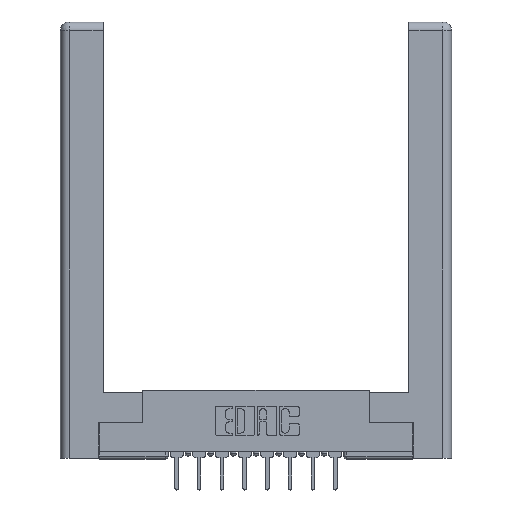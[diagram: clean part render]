
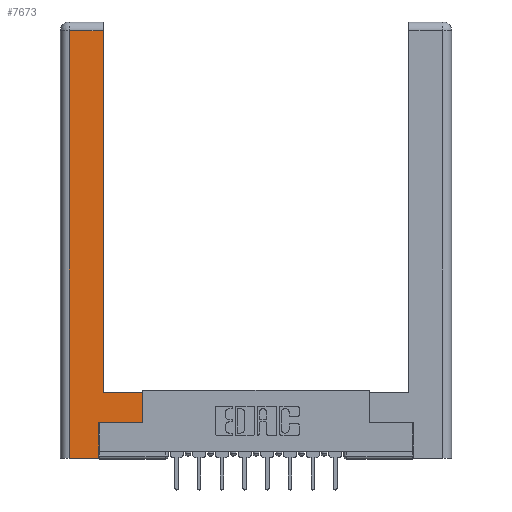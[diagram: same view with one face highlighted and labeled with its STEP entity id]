
A CAD part, top view. The second image highlights one B-rep face of the part: STEP entity #7673.
In plain terms, the highlighted planar face has unit normal (0, 0, 1).
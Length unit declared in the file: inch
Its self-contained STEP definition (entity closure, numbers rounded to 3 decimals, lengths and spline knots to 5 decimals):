
#47 = ORIENTED_EDGE ( 'NONE', *, *, #10888, .T. ) ;
#483 = VECTOR ( 'NONE', #7286, 39.37008 ) ;
#524 = VERTEX_POINT ( 'NONE', #10340 ) ;
#594 = VERTEX_POINT ( 'NONE', #11713 ) ;
#708 = LINE ( 'NONE', #6021, #10337 ) ;
#760 = CARTESIAN_POINT ( 'NONE',  ( 0., 0., 0. ) ) ;
#1495 = VERTEX_POINT ( 'NONE', #9844 ) ;
#2049 = CARTESIAN_POINT ( 'NONE',  ( 0.0615, 2.94, 0. ) ) ;
#2069 = EDGE_LOOP ( 'NONE', ( #8152, #12414, #2658, #11742, #12589, #47, #9394, #8304 ) ) ;
#2121 = VERTEX_POINT ( 'NONE', #3643 ) ;
#2325 = LINE ( 'NONE', #9720, #8539 ) ;
#2658 = ORIENTED_EDGE ( 'NONE', *, *, #9716, .T. ) ;
#2790 = EDGE_CURVE ( 'NONE', #594, #1495, #7426, .T. ) ;
#2829 = DIRECTION ( 'NONE',  ( 1., 0., 0. ) ) ;
#3191 = VERTEX_POINT ( 'NONE', #11083 ) ;
#3304 = EDGE_CURVE ( 'NONE', #11582, #524, #5072, .T. ) ;
#3446 = CARTESIAN_POINT ( 'NONE',  ( 0.565, 0.45, 0. ) ) ;
#3519 = VERTEX_POINT ( 'NONE', #10596 ) ;
#3635 = VECTOR ( 'NONE', #7417, 39.37008 ) ;
#3643 = CARTESIAN_POINT ( 'NONE',  ( 0.295, 0.45, 0. ) ) ;
#3862 = CARTESIAN_POINT ( 'NONE',  ( 0.565, 0.245, 0. ) ) ;
#4245 = LINE ( 'NONE', #9572, #8725 ) ;
#4679 = VECTOR ( 'NONE', #11645, 39.37008 ) ;
#4743 = CARTESIAN_POINT ( 'NONE',  ( 0.565, 0.245, 0. ) ) ;
#4900 = VECTOR ( 'NONE', #10781, 39.37008 ) ;
#4964 = PLANE ( 'NONE',  #10704 ) ;
#5072 = LINE ( 'NONE', #9495, #483 ) ;
#5201 = EDGE_CURVE ( 'NONE', #12874, #3191, #11887, .T. ) ;
#6021 = CARTESIAN_POINT ( 'NONE',  ( 0.295, 3., 0. ) ) ;
#7286 = DIRECTION ( 'NONE',  ( 1., 0., 0. ) ) ;
#7417 = DIRECTION ( 'NONE',  ( -1., 0., 0. ) ) ;
#7426 = LINE ( 'NONE', #2049, #4679 ) ;
#7554 = DIRECTION ( 'NONE',  ( 0., 1., 0. ) ) ;
#7673 = ADVANCED_FACE ( 'NONE', ( #11255 ), #4964, .F. ) ;
#8152 = ORIENTED_EDGE ( 'NONE', *, *, #12178, .T. ) ;
#8190 = EDGE_CURVE ( 'NONE', #3191, #2121, #9499, .T. ) ;
#8304 = ORIENTED_EDGE ( 'NONE', *, *, #8190, .T. ) ;
#8539 = VECTOR ( 'NONE', #11728, 39.37008 ) ;
#8725 = VECTOR ( 'NONE', #7554, 39.37008 ) ;
#9117 = DIRECTION ( 'NONE',  ( -1., 0., 0. ) ) ;
#9336 = DIRECTION ( 'NONE',  ( 0., 1., 0. ) ) ;
#9394 = ORIENTED_EDGE ( 'NONE', *, *, #5201, .T. ) ;
#9495 = CARTESIAN_POINT ( 'NONE',  ( 0.265, 0., 0. ) ) ;
#9499 = LINE ( 'NONE', #12817, #3635 ) ;
#9572 = CARTESIAN_POINT ( 'NONE',  ( 0.265, 0.245, 0. ) ) ;
#9716 = EDGE_CURVE ( 'NONE', #1495, #11582, #2325, .T. ) ;
#9720 = CARTESIAN_POINT ( 'NONE',  ( 0.0615, 0., 0. ) ) ;
#9844 = CARTESIAN_POINT ( 'NONE',  ( 0.0615, 2.94, 0. ) ) ;
#10013 = DIRECTION ( 'NONE',  ( 0., 0., -1. ) ) ;
#10207 = EDGE_CURVE ( 'NONE', #524, #3519, #4245, .T. ) ;
#10304 = VECTOR ( 'NONE', #2829, 39.37008 ) ;
#10337 = VECTOR ( 'NONE', #9336, 39.37008 ) ;
#10340 = CARTESIAN_POINT ( 'NONE',  ( 0.265, 0., 0. ) ) ;
#10596 = CARTESIAN_POINT ( 'NONE',  ( 0.265, 0.245, 0. ) ) ;
#10704 = AXIS2_PLACEMENT_3D ( 'NONE', #760, #10013, #9117 ) ;
#10781 = DIRECTION ( 'NONE',  ( 0., 1., 0. ) ) ;
#10888 = EDGE_CURVE ( 'NONE', #3519, #12874, #13562, .T. ) ;
#11083 = CARTESIAN_POINT ( 'NONE',  ( 0.565, 0.45, 0. ) ) ;
#11255 = FACE_OUTER_BOUND ( 'NONE', #2069, .T. ) ;
#11582 = VERTEX_POINT ( 'NONE', #12962 ) ;
#11645 = DIRECTION ( 'NONE',  ( -1., 0., 0. ) ) ;
#11713 = CARTESIAN_POINT ( 'NONE',  ( 0.295, 2.94, 0. ) ) ;
#11728 = DIRECTION ( 'NONE',  ( 0., -1., 0. ) ) ;
#11742 = ORIENTED_EDGE ( 'NONE', *, *, #3304, .T. ) ;
#11887 = LINE ( 'NONE', #3446, #4900 ) ;
#12178 = EDGE_CURVE ( 'NONE', #2121, #594, #708, .T. ) ;
#12414 = ORIENTED_EDGE ( 'NONE', *, *, #2790, .T. ) ;
#12589 = ORIENTED_EDGE ( 'NONE', *, *, #10207, .T. ) ;
#12817 = CARTESIAN_POINT ( 'NONE',  ( 0.295, 0.45, 0. ) ) ;
#12874 = VERTEX_POINT ( 'NONE', #4743 ) ;
#12962 = CARTESIAN_POINT ( 'NONE',  ( 0.0615, 0., 0. ) ) ;
#13562 = LINE ( 'NONE', #3862, #10304 ) ;
